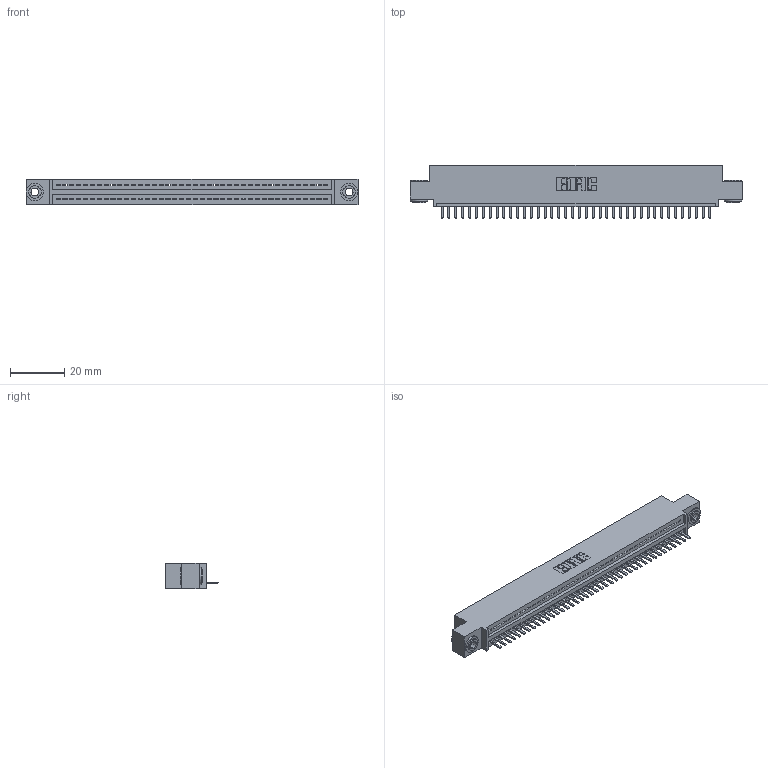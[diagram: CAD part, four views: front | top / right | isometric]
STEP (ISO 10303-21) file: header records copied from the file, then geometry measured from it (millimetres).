
FILE_DESCRIPTION (( 'STEP AP203' ), '1' );
FILE_NAME ('395-040-520-403.STEP', '2018-11-14T15:18:32', ( '' ), ( '' ), 'SwSTEP 2.0', 'SolidWorks 2016', '' );
FILE_SCHEMA (( 'CONFIG_CONTROL_DESIGN' ));
Length unit declared in the file: inch
Products named in the file (4): 395-040-520-403; 345-250-002_345-250-002-102; 345 Part_0.110 Offset - 0.156 Dia-TH; 345-292-001_345-293-120
Assembly tree (43 placements, depth 2):
  395-040-520-403
    345 Part_0.110 Offset - 0.156 Dia-TH
    345-292-001_345-293-120  x40
    345-250-002_345-250-002-102  x2
Bounding box: 122.81 x 19.68 x 9.4 mm (x, y, z)
Volume: 11479.1 mm3; surface area: 15147.5 mm2
Topology: 43 solids, 43 shells, 2648 faces, 7789 edges, 5082 vertices
Faces by surface type: plane 1774, cylinder 866, cone 8
Entity records: 31270 total; most frequent: CARTESIAN_POINT 5407, ORIENTED_EDGE 5362, DIRECTION 4743, EDGE_CURVE 2681, LINE 2361, VECTOR 2361, VERTEX_POINT 1782, AXIS2_PLACEMENT_3D 1191
